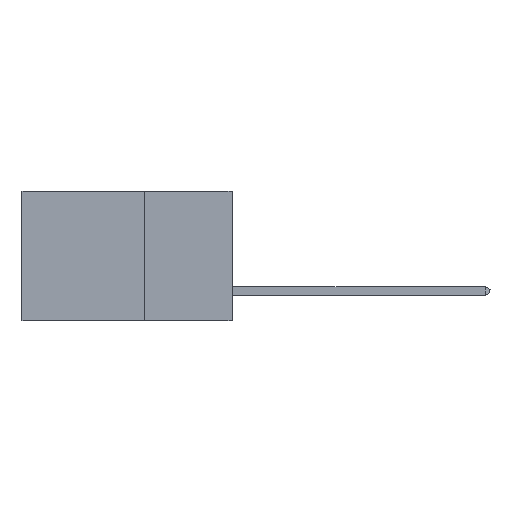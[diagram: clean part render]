
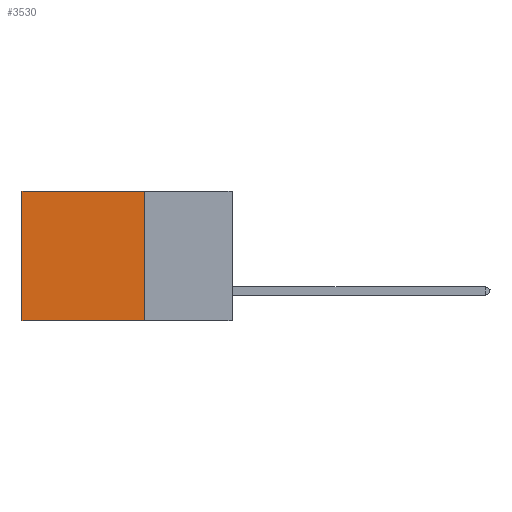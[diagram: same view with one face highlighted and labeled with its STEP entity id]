
A CAD part, left-side view. The second image highlights one B-rep face of the part: STEP entity #3530.
In plain terms, the highlighted planar face has unit normal (-1, 0, 0).
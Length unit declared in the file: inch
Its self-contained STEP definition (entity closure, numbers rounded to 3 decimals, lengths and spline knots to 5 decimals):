
#337 = VERTEX_POINT ( 'NONE', #18688 ) ;
#400 = LINE ( 'NONE', #1763, #4550 ) ;
#1591 = FACE_OUTER_BOUND ( 'NONE', #19889, .T. ) ;
#1679 = EDGE_CURVE ( 'NONE', #2843, #337, #11264, .T. ) ;
#1763 = CARTESIAN_POINT ( 'NONE',  ( 0.2875, 0.25, 0. ) ) ;
#2843 = VERTEX_POINT ( 'NONE', #16566 ) ;
#3160 = ORIENTED_EDGE ( 'NONE', *, *, #8266, .T. ) ;
#3282 = VERTEX_POINT ( 'NONE', #9230 ) ;
#3530 = ADVANCED_FACE ( 'NONE', ( #1591 ), #12826, .F. ) ;
#4550 = VECTOR ( 'NONE', #7567, 39.37008 ) ;
#7511 = ORIENTED_EDGE ( 'NONE', *, *, #20475, .F. ) ;
#7567 = DIRECTION ( 'NONE',  ( 0., 0., -1. ) ) ;
#8266 = EDGE_CURVE ( 'NONE', #3282, #2843, #20598, .T. ) ;
#8464 = CARTESIAN_POINT ( 'NONE',  ( 0.2875, 0.25, 0. ) ) ;
#9043 = VECTOR ( 'NONE', #22419, 39.37008 ) ;
#9230 = CARTESIAN_POINT ( 'NONE',  ( 0.2875, 0.25, 0. ) ) ;
#9232 = AXIS2_PLACEMENT_3D ( 'NONE', #8464, #18914, #14688 ) ;
#9370 = ORIENTED_EDGE ( 'NONE', *, *, #1679, .T. ) ;
#11198 = CARTESIAN_POINT ( 'NONE',  ( 0.2875, 0.25, 0. ) ) ;
#11264 = LINE ( 'NONE', #18210, #9043 ) ;
#12456 = VERTEX_POINT ( 'NONE', #23823 ) ;
#12826 = PLANE ( 'NONE',  #9232 ) ;
#14318 = VECTOR ( 'NONE', #17552, 39.37008 ) ;
#14688 = DIRECTION ( 'NONE',  ( 0., 0., -1. ) ) ;
#15868 = CARTESIAN_POINT ( 'NONE',  ( 0.2875, 0.25, -0.37 ) ) ;
#16566 = CARTESIAN_POINT ( 'NONE',  ( 0.2875, 0.6, 0. ) ) ;
#17478 = DIRECTION ( 'NONE',  ( 0., 1., 0. ) ) ;
#17552 = DIRECTION ( 'NONE',  ( 0., 1., 0. ) ) ;
#18210 = CARTESIAN_POINT ( 'NONE',  ( 0.2875, 0.6, 0. ) ) ;
#18688 = CARTESIAN_POINT ( 'NONE',  ( 0.2875, 0.6, -0.37 ) ) ;
#18742 = EDGE_CURVE ( 'NONE', #3282, #12456, #400, .T. ) ;
#18914 = DIRECTION ( 'NONE',  ( 1., 0., 0. ) ) ;
#19889 = EDGE_LOOP ( 'NONE', ( #9370, #7511, #20234, #3160 ) ) ;
#20234 = ORIENTED_EDGE ( 'NONE', *, *, #18742, .F. ) ;
#20475 = EDGE_CURVE ( 'NONE', #12456, #337, #22902, .T. ) ;
#20598 = LINE ( 'NONE', #11198, #21876 ) ;
#21876 = VECTOR ( 'NONE', #17478, 39.37008 ) ;
#22419 = DIRECTION ( 'NONE',  ( 0., 0., -1. ) ) ;
#22902 = LINE ( 'NONE', #15868, #14318 ) ;
#23823 = CARTESIAN_POINT ( 'NONE',  ( 0.2875, 0.25, -0.37 ) ) ;
